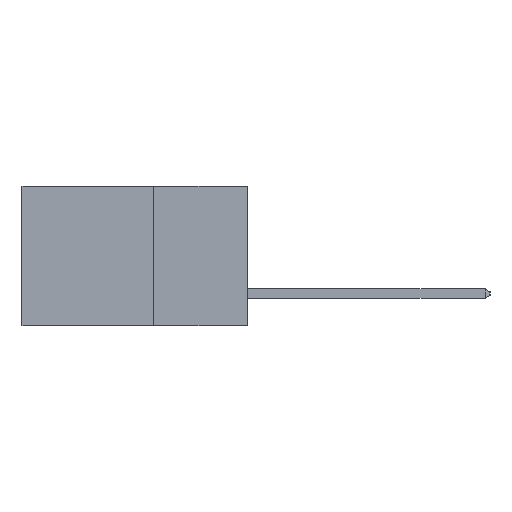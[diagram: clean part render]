
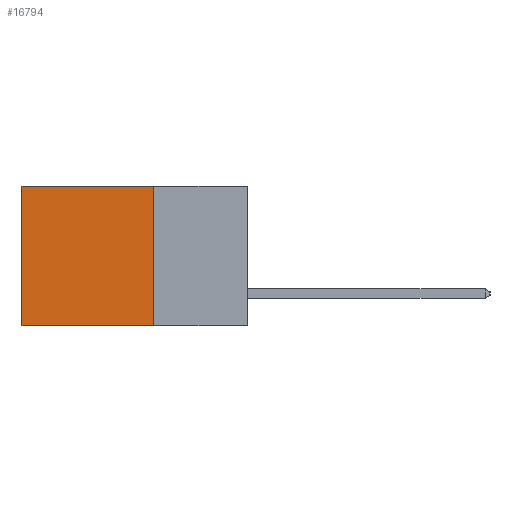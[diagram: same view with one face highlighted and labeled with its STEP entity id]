
A CAD part, left-side view. The second image highlights one B-rep face of the part: STEP entity #16794.
In plain terms, the highlighted planar face has unit normal (-1, 0, 0).
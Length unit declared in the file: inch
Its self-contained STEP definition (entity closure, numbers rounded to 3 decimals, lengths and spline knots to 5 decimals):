
#151 = CARTESIAN_POINT ( 'NONE',  ( 0.2615, 0.25, -0.37 ) ) ;
#1078 = VERTEX_POINT ( 'NONE', #23207 ) ;
#1156 = VERTEX_POINT ( 'NONE', #2929 ) ;
#1536 = DIRECTION ( 'NONE',  ( 0., 1., 0. ) ) ;
#1623 = CARTESIAN_POINT ( 'NONE',  ( 0.2615, 0.25, 0. ) ) ;
#1957 = VERTEX_POINT ( 'NONE', #19577 ) ;
#2132 = LINE ( 'NONE', #13705, #22370 ) ;
#2929 = CARTESIAN_POINT ( 'NONE',  ( 0.2615, 0.25, 0. ) ) ;
#4130 = DIRECTION ( 'NONE',  ( 1., 0., 0. ) ) ;
#4493 = VECTOR ( 'NONE', #17925, 39.37008 ) ;
#7517 = AXIS2_PLACEMENT_3D ( 'NONE', #16328, #4130, #18324 ) ;
#8728 = VERTEX_POINT ( 'NONE', #24774 ) ;
#9152 = EDGE_LOOP ( 'NONE', ( #22319, #21148, #15511, #19082 ) ) ;
#9906 = LINE ( 'NONE', #19940, #4493 ) ;
#11326 = EDGE_CURVE ( 'NONE', #1156, #1078, #22500, .T. ) ;
#13705 = CARTESIAN_POINT ( 'NONE',  ( 0.2615, 0.6, -0.37 ) ) ;
#15511 = ORIENTED_EDGE ( 'NONE', *, *, #23184, .F. ) ;
#15698 = LINE ( 'NONE', #151, #25031 ) ;
#16328 = CARTESIAN_POINT ( 'NONE',  ( 0.2615, 0.25, -0.37 ) ) ;
#16521 = DIRECTION ( 'NONE',  ( 0., 1., 0. ) ) ;
#16794 = ADVANCED_FACE ( 'NONE', ( #18576 ), #26186, .F. ) ;
#17925 = DIRECTION ( 'NONE',  ( 0., 0., -1. ) ) ;
#18324 = DIRECTION ( 'NONE',  ( 0., 0., -1. ) ) ;
#18576 = FACE_OUTER_BOUND ( 'NONE', #9152, .T. ) ;
#19082 = ORIENTED_EDGE ( 'NONE', *, *, #11326, .T. ) ;
#19577 = CARTESIAN_POINT ( 'NONE',  ( 0.2615, 0.6, -0.37 ) ) ;
#19940 = CARTESIAN_POINT ( 'NONE',  ( 0.2615, 0.25, -0.37 ) ) ;
#21148 = ORIENTED_EDGE ( 'NONE', *, *, #22191, .F. ) ;
#21699 = DIRECTION ( 'NONE',  ( 0., 0., -1. ) ) ;
#22191 = EDGE_CURVE ( 'NONE', #8728, #1957, #15698, .T. ) ;
#22319 = ORIENTED_EDGE ( 'NONE', *, *, #25603, .T. ) ;
#22370 = VECTOR ( 'NONE', #21699, 39.37008 ) ;
#22500 = LINE ( 'NONE', #1623, #23112 ) ;
#23112 = VECTOR ( 'NONE', #1536, 39.37008 ) ;
#23184 = EDGE_CURVE ( 'NONE', #1156, #8728, #9906, .T. ) ;
#23207 = CARTESIAN_POINT ( 'NONE',  ( 0.2615, 0.6, 0. ) ) ;
#24774 = CARTESIAN_POINT ( 'NONE',  ( 0.2615, 0.25, -0.37 ) ) ;
#25031 = VECTOR ( 'NONE', #16521, 39.37008 ) ;
#25603 = EDGE_CURVE ( 'NONE', #1078, #1957, #2132, .T. ) ;
#26186 = PLANE ( 'NONE',  #7517 ) ;
